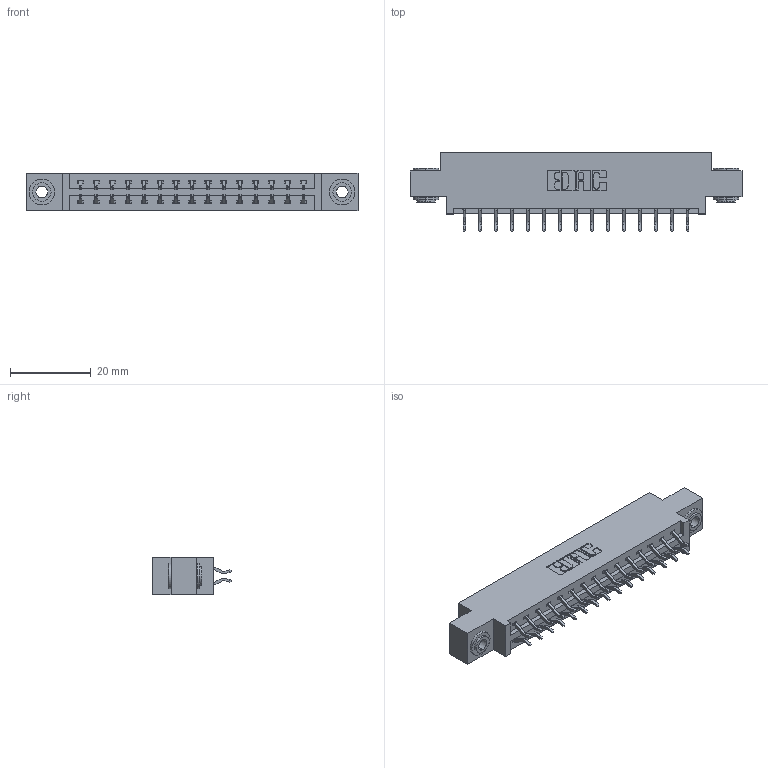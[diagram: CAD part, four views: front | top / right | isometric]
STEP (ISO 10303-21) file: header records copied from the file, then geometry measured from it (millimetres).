
FILE_DESCRIPTION (( 'STEP AP203' ), '1' );
FILE_NAME ('387-030-556-803.STEP', '2018-09-18T03:12:06', ( '' ), ( '' ), 'SwSTEP 2.0', 'SolidWorks 2016', '' );
FILE_SCHEMA (( 'CONFIG_CONTROL_DESIGN' ));
Length unit declared in the file: inch
Products named in the file (4): 337 Part_0.170 Offset - 0.156 Dia-TH; 345-292-001_556 Tail; 345-250-002_345-250-002-102; 387-030-556-803
Assembly tree (33 placements, depth 2):
  387-030-556-803
    337 Part_0.170 Offset - 0.156 Dia-TH
    345-292-001_556 Tail  x30
    345-250-002_345-250-002-102  x2
Bounding box: 82.45 x 19.57 x 9.4 mm (x, y, z)
Volume: 8230.4 mm3; surface area: 9342.8 mm2
Topology: 33 solids, 33 shells, 1956 faces, 5769 edges, 3802 vertices
Faces by surface type: plane 1344, cylinder 604, cone 8
Entity records: 16124 total; most frequent: CARTESIAN_POINT 2729, ORIENTED_EDGE 2646, DIRECTION 2393, EDGE_CURVE 1323, VECTOR 1163, LINE 1163, VERTEX_POINT 878, AXIS2_PLACEMENT_3D 615
